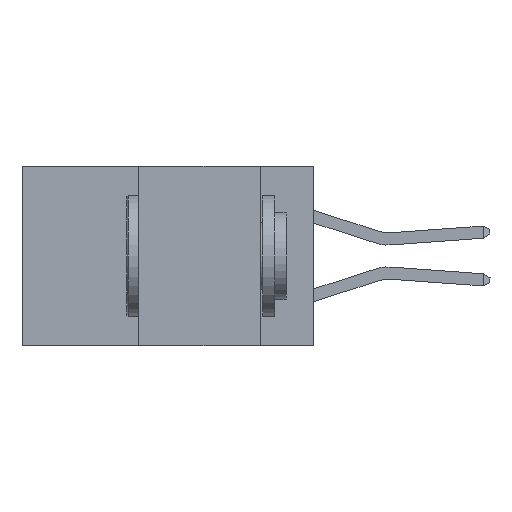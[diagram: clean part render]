
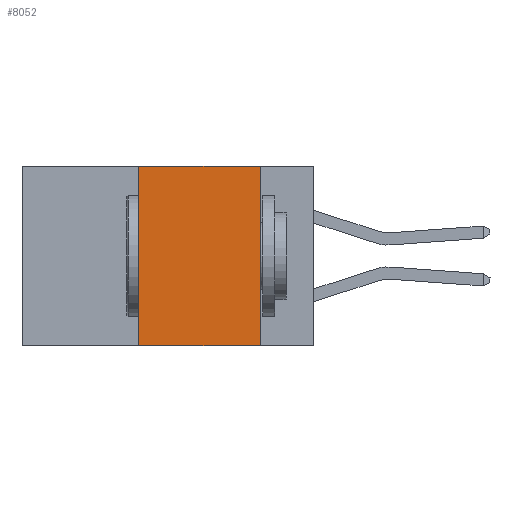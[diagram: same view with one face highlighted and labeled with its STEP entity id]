
A CAD part, left-side view. The second image highlights one B-rep face of the part: STEP entity #8052.
In plain terms, the highlighted planar face has unit normal (-1, 0, 0).
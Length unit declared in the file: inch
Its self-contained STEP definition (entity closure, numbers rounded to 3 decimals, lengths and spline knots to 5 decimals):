
#62 = VERTEX_POINT ( 'NONE', #10061 ) ;
#288 = CARTESIAN_POINT ( 'NONE',  ( 0., 0.36, -0.37 ) ) ;
#464 = PLANE ( 'NONE',  #1396 ) ;
#620 = FACE_OUTER_BOUND ( 'NONE', #1548, .T. ) ;
#1396 = AXIS2_PLACEMENT_3D ( 'NONE', #5670, #7662, #1515 ) ;
#1515 = DIRECTION ( 'NONE',  ( 0., 0., -1. ) ) ;
#1548 = EDGE_LOOP ( 'NONE', ( #6150, #6348, #6611, #7288 ) ) ;
#1972 = LINE ( 'NONE', #5604, #9760 ) ;
#2837 = LINE ( 'NONE', #6158, #9644 ) ;
#3328 = EDGE_CURVE ( 'NONE', #10756, #62, #7049, .T. ) ;
#3796 = EDGE_CURVE ( 'NONE', #10756, #8879, #2837, .T. ) ;
#3819 = EDGE_CURVE ( 'NONE', #10384, #62, #4262, .T. ) ;
#4262 = LINE ( 'NONE', #5894, #6749 ) ;
#4275 = VECTOR ( 'NONE', #9799, 39.37008 ) ;
#5141 = CARTESIAN_POINT ( 'NONE',  ( 0., 0.11, 0. ) ) ;
#5540 = CARTESIAN_POINT ( 'NONE',  ( 0., 0.36, 0. ) ) ;
#5604 = CARTESIAN_POINT ( 'NONE',  ( 0., 0.6, 0. ) ) ;
#5670 = CARTESIAN_POINT ( 'NONE',  ( 0., 0.6, 0. ) ) ;
#5747 = DIRECTION ( 'NONE',  ( 0., 0., -1. ) ) ;
#5894 = CARTESIAN_POINT ( 'NONE',  ( 0., 0.11, 0. ) ) ;
#6079 = DIRECTION ( 'NONE',  ( 0., 0., 1. ) ) ;
#6150 = ORIENTED_EDGE ( 'NONE', *, *, #3819, .F. ) ;
#6158 = CARTESIAN_POINT ( 'NONE',  ( 0., 0.36, 0. ) ) ;
#6348 = ORIENTED_EDGE ( 'NONE', *, *, #12612, .F. ) ;
#6611 = ORIENTED_EDGE ( 'NONE', *, *, #3796, .F. ) ;
#6749 = VECTOR ( 'NONE', #5747, 39.37008 ) ;
#7049 = LINE ( 'NONE', #9884, #4275 ) ;
#7288 = ORIENTED_EDGE ( 'NONE', *, *, #3328, .T. ) ;
#7662 = DIRECTION ( 'NONE',  ( 1., 0., 0. ) ) ;
#8052 = ADVANCED_FACE ( 'NONE', ( #620 ), #464, .F. ) ;
#8879 = VERTEX_POINT ( 'NONE', #5540 ) ;
#9644 = VECTOR ( 'NONE', #6079, 39.37008 ) ;
#9760 = VECTOR ( 'NONE', #11485, 39.37008 ) ;
#9799 = DIRECTION ( 'NONE',  ( 0., -1., 0. ) ) ;
#9884 = CARTESIAN_POINT ( 'NONE',  ( 0., 0.6, -0.37 ) ) ;
#10061 = CARTESIAN_POINT ( 'NONE',  ( 0., 0.11, -0.37 ) ) ;
#10384 = VERTEX_POINT ( 'NONE', #5141 ) ;
#10756 = VERTEX_POINT ( 'NONE', #288 ) ;
#11485 = DIRECTION ( 'NONE',  ( 0., -1., 0. ) ) ;
#12612 = EDGE_CURVE ( 'NONE', #8879, #10384, #1972, .T. ) ;
